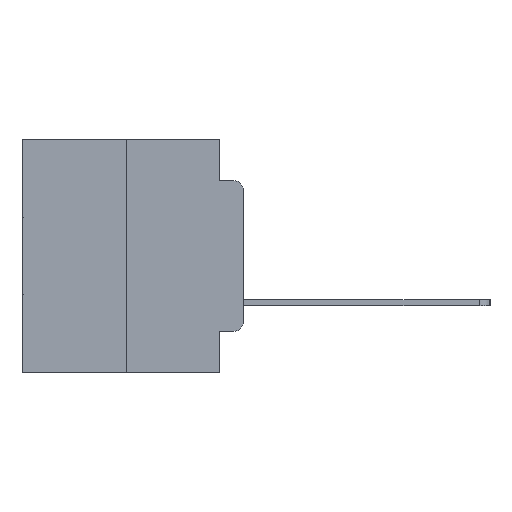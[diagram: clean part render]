
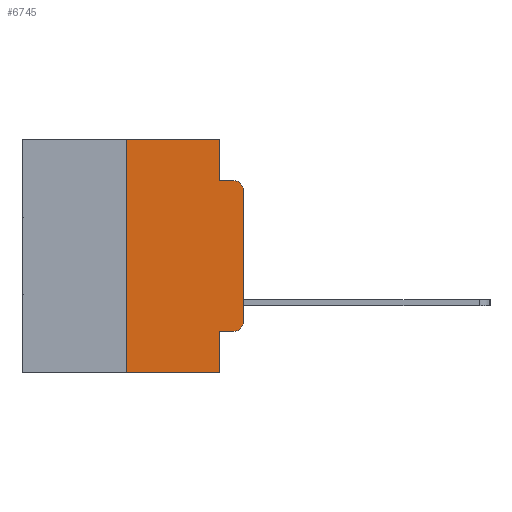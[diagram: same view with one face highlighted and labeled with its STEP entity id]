
A CAD part, left-side view. The second image highlights one B-rep face of the part: STEP entity #6745.
In plain terms, the highlighted planar face has unit normal (-1, 0, 0).
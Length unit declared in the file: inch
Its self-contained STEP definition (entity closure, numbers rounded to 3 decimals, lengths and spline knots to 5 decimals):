
#207 = ORIENTED_EDGE ( 'NONE', *, *, #2668, .F. ) ;
#401 = ORIENTED_EDGE ( 'NONE', *, *, #22585, .T. ) ;
#609 = VERTEX_POINT ( 'NONE', #11912 ) ;
#1916 = LINE ( 'NONE', #12312, #12843 ) ;
#1968 = VERTEX_POINT ( 'NONE', #23639 ) ;
#2125 = DIRECTION ( 'NONE',  ( 0., -1., 0. ) ) ;
#2627 = EDGE_CURVE ( 'NONE', #16076, #10711, #16581, .T. ) ;
#2668 = EDGE_CURVE ( 'NONE', #6090, #609, #15162, .T. ) ;
#2838 = CARTESIAN_POINT ( 'NONE',  ( 0., 0.051, 0. ) ) ;
#3412 = ORIENTED_EDGE ( 'NONE', *, *, #5233, .T. ) ;
#3564 = EDGE_LOOP ( 'NONE', ( #401, #3412, #5204, #27972, #29021, #207, #13653, #13709, #12324, #20872 ) ) ;
#3974 = VERTEX_POINT ( 'NONE', #4832 ) ;
#4832 = CARTESIAN_POINT ( 'NONE',  ( 0., 0., -0.1085 ) ) ;
#5204 = ORIENTED_EDGE ( 'NONE', *, *, #20097, .F. ) ;
#5233 = EDGE_CURVE ( 'NONE', #3974, #25980, #12171, .T. ) ;
#5909 = LINE ( 'NONE', #27540, #23523 ) ;
#6090 = VERTEX_POINT ( 'NONE', #29591 ) ;
#6196 = VECTOR ( 'NONE', #25081, 39.37008 ) ;
#6462 = LINE ( 'NONE', #29647, #18027 ) ;
#6745 = ADVANCED_FACE ( 'NONE', ( #16677 ), #22820, .F. ) ;
#6820 = CARTESIAN_POINT ( 'NONE',  ( 0., 0.051, 0. ) ) ;
#8587 = LINE ( 'NONE', #26158, #20100 ) ;
#8830 = CARTESIAN_POINT ( 'NONE',  ( 0., 0., -0.3915 ) ) ;
#9018 = VECTOR ( 'NONE', #15908, 39.37008 ) ;
#9162 = DIRECTION ( 'NONE',  ( 0., 0., -1. ) ) ;
#9807 = LINE ( 'NONE', #26156, #26651 ) ;
#9868 = CARTESIAN_POINT ( 'NONE',  ( 0., 0.02, -0.3915 ) ) ;
#10135 = DIRECTION ( 'NONE',  ( 0., 0., -1. ) ) ;
#10657 = AXIS2_PLACEMENT_3D ( 'NONE', #9868, #25910, #12215 ) ;
#10711 = VERTEX_POINT ( 'NONE', #8830 ) ;
#11755 = DIRECTION ( 'NONE',  ( -1., 0., 0. ) ) ;
#11912 = CARTESIAN_POINT ( 'NONE',  ( 0., 0.25, 0. ) ) ;
#12171 = CIRCLE ( 'NONE', #18417, 0.02 ) ;
#12213 = LINE ( 'NONE', #6820, #23648 ) ;
#12215 = DIRECTION ( 'NONE',  ( 0., 0., -1. ) ) ;
#12279 = CARTESIAN_POINT ( 'NONE',  ( 0., 0.02, -0.4115 ) ) ;
#12312 = CARTESIAN_POINT ( 'NONE',  ( 0., 0.051, -0.0885 ) ) ;
#12324 = ORIENTED_EDGE ( 'NONE', *, *, #26566, .T. ) ;
#12843 = VECTOR ( 'NONE', #21397, 39.37008 ) ;
#13653 = ORIENTED_EDGE ( 'NONE', *, *, #20579, .T. ) ;
#13709 = ORIENTED_EDGE ( 'NONE', *, *, #27337, .F. ) ;
#13891 = CARTESIAN_POINT ( 'NONE',  ( 0., 0.051, -0.4115 ) ) ;
#15162 = LINE ( 'NONE', #18235, #9018 ) ;
#15908 = DIRECTION ( 'NONE',  ( 0., 0., 1. ) ) ;
#16010 = DIRECTION ( 'NONE',  ( 0., 0., -1. ) ) ;
#16076 = VERTEX_POINT ( 'NONE', #12279 ) ;
#16581 = CIRCLE ( 'NONE', #10657, 0.02 ) ;
#16677 = FACE_OUTER_BOUND ( 'NONE', #3564, .T. ) ;
#18027 = VECTOR ( 'NONE', #2125, 39.37008 ) ;
#18235 = CARTESIAN_POINT ( 'NONE',  ( 0., 0.25, 0. ) ) ;
#18417 = AXIS2_PLACEMENT_3D ( 'NONE', #25458, #11755, #27733 ) ;
#20097 = EDGE_CURVE ( 'NONE', #1968, #25980, #1916, .T. ) ;
#20100 = VECTOR ( 'NONE', #10135, 39.37008 ) ;
#20503 = CARTESIAN_POINT ( 'NONE',  ( 0., 0.051, -0.5 ) ) ;
#20579 = EDGE_CURVE ( 'NONE', #6090, #28880, #5909, .T. ) ;
#20872 = ORIENTED_EDGE ( 'NONE', *, *, #2627, .T. ) ;
#21397 = DIRECTION ( 'NONE',  ( 0., -1., 0. ) ) ;
#22278 = EDGE_CURVE ( 'NONE', #609, #26745, #23819, .T. ) ;
#22585 = EDGE_CURVE ( 'NONE', #10711, #3974, #9807, .T. ) ;
#22785 = CARTESIAN_POINT ( 'NONE',  ( 0., 0.473, 0. ) ) ;
#22820 = PLANE ( 'NONE',  #23207 ) ;
#23207 = AXIS2_PLACEMENT_3D ( 'NONE', #27388, #29654, #16010 ) ;
#23523 = VECTOR ( 'NONE', #29824, 39.37008 ) ;
#23639 = CARTESIAN_POINT ( 'NONE',  ( 0., 0.051, -0.0885 ) ) ;
#23648 = VECTOR ( 'NONE', #9162, 39.37008 ) ;
#23819 = LINE ( 'NONE', #22785, #6196 ) ;
#25081 = DIRECTION ( 'NONE',  ( 0., -1., 0. ) ) ;
#25326 = CARTESIAN_POINT ( 'NONE',  ( 0., 0.02, -0.0885 ) ) ;
#25458 = CARTESIAN_POINT ( 'NONE',  ( 0., 0.02, -0.1085 ) ) ;
#25910 = DIRECTION ( 'NONE',  ( -1., 0., 0. ) ) ;
#25980 = VERTEX_POINT ( 'NONE', #25326 ) ;
#26156 = CARTESIAN_POINT ( 'NONE',  ( 0., 0., 0. ) ) ;
#26158 = CARTESIAN_POINT ( 'NONE',  ( 0., 0.051, 0. ) ) ;
#26566 = EDGE_CURVE ( 'NONE', #28360, #16076, #6462, .T. ) ;
#26651 = VECTOR ( 'NONE', #28430, 39.37008 ) ;
#26745 = VERTEX_POINT ( 'NONE', #2838 ) ;
#27337 = EDGE_CURVE ( 'NONE', #28360, #28880, #8587, .T. ) ;
#27388 = CARTESIAN_POINT ( 'NONE',  ( 0., 0.473, 0. ) ) ;
#27540 = CARTESIAN_POINT ( 'NONE',  ( 0., 0.473, -0.5 ) ) ;
#27733 = DIRECTION ( 'NONE',  ( 0., 0., -1. ) ) ;
#27972 = ORIENTED_EDGE ( 'NONE', *, *, #28291, .F. ) ;
#28291 = EDGE_CURVE ( 'NONE', #26745, #1968, #12213, .T. ) ;
#28360 = VERTEX_POINT ( 'NONE', #13891 ) ;
#28430 = DIRECTION ( 'NONE',  ( 0., 0., 1. ) ) ;
#28880 = VERTEX_POINT ( 'NONE', #20503 ) ;
#29021 = ORIENTED_EDGE ( 'NONE', *, *, #22278, .F. ) ;
#29591 = CARTESIAN_POINT ( 'NONE',  ( 0., 0.25, -0.5 ) ) ;
#29647 = CARTESIAN_POINT ( 'NONE',  ( 0., 0.051, -0.4115 ) ) ;
#29654 = DIRECTION ( 'NONE',  ( 1., 0., 0. ) ) ;
#29824 = DIRECTION ( 'NONE',  ( 0., -1., 0. ) ) ;
